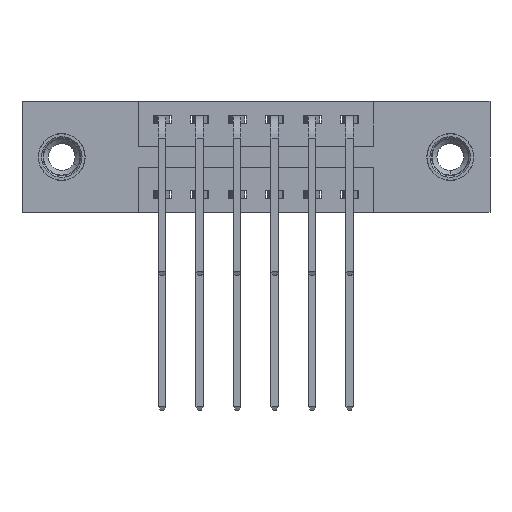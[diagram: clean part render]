
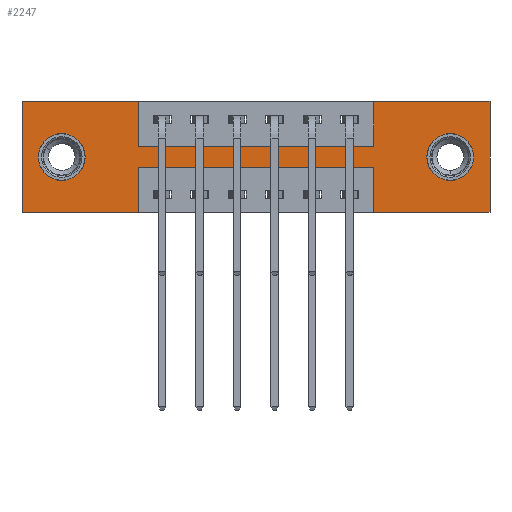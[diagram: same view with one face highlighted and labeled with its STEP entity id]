
A CAD part, front view. The second image highlights one B-rep face of the part: STEP entity #2247.
In plain terms, the highlighted planar face has unit normal (0, -1, 0).
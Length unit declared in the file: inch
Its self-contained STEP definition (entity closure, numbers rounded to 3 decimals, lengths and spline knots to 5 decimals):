
#42 = VERTEX_POINT ( 'NONE', #2623 ) ;
#102 = CARTESIAN_POINT ( 'NONE',  ( 1.4275, 0., -0.263 ) ) ;
#105 = ORIENTED_EDGE ( 'NONE', *, *, #3192, .F. ) ;
#121 = DIRECTION ( 'NONE',  ( 0., 0., -1. ) ) ;
#225 = CARTESIAN_POINT ( 'NONE',  ( 0., 0., 0. ) ) ;
#446 = CARTESIAN_POINT ( 'NONE',  ( 1.1725, 0., -0.37 ) ) ;
#526 = CARTESIAN_POINT ( 'NONE',  ( 0., 0., -0.37 ) ) ;
#544 = ORIENTED_EDGE ( 'NONE', *, *, #9212, .F. ) ;
#617 = ORIENTED_EDGE ( 'NONE', *, *, #5283, .F. ) ;
#626 = EDGE_CURVE ( 'NONE', #9823, #6591, #4002, .T. ) ;
#648 = VECTOR ( 'NONE', #1147, 39.37008 ) ;
#671 = AXIS2_PLACEMENT_3D ( 'NONE', #6473, #2868, #6435 ) ;
#1073 = DIRECTION ( 'NONE',  ( 1., 0., 0. ) ) ;
#1147 = DIRECTION ( 'NONE',  ( 0., 0., 1. ) ) ;
#1294 = EDGE_LOOP ( 'NONE', ( #617, #9598, #105, #4870, #7537, #4949, #3419, #544, #4352, #2203, #3891, #4409 ) ) ;
#1433 = CARTESIAN_POINT ( 'NONE',  ( 0.3875, 0., -0.37 ) ) ;
#1494 = LINE ( 'NONE', #11450, #3079 ) ;
#1506 = AXIS2_PLACEMENT_3D ( 'NONE', #7502, #6528, #4697 ) ;
#1885 = CARTESIAN_POINT ( 'NONE',  ( 0., 0., -0.37 ) ) ;
#2133 = AXIS2_PLACEMENT_3D ( 'NONE', #4694, #5673, #11016 ) ;
#2203 = ORIENTED_EDGE ( 'NONE', *, *, #8036, .F. ) ;
#2247 = ADVANCED_FACE ( 'NONE', ( #11677, #4725, #2288 ), #10993, .T. ) ;
#2263 = CARTESIAN_POINT ( 'NONE',  ( 0.3875, 0., -0.22 ) ) ;
#2288 = FACE_OUTER_BOUND ( 'NONE', #1294, .T. ) ;
#2499 = VECTOR ( 'NONE', #7907, 39.37008 ) ;
#2503 = LINE ( 'NONE', #5610, #10180 ) ;
#2623 = CARTESIAN_POINT ( 'NONE',  ( 0.1325, 0., -0.263 ) ) ;
#2700 = DIRECTION ( 'NONE',  ( 0., 1., 0. ) ) ;
#2743 = CARTESIAN_POINT ( 'NONE',  ( 0., 0., 0. ) ) ;
#2868 = DIRECTION ( 'NONE',  ( 0., 1., 0. ) ) ;
#2912 = VECTOR ( 'NONE', #4324, 39.37008 ) ;
#2934 = LINE ( 'NONE', #225, #8328 ) ;
#3079 = VECTOR ( 'NONE', #7864, 39.37008 ) ;
#3098 = AXIS2_PLACEMENT_3D ( 'NONE', #5759, #9308, #121 ) ;
#3192 = EDGE_CURVE ( 'NONE', #3302, #3218, #6525, .T. ) ;
#3218 = VERTEX_POINT ( 'NONE', #11252 ) ;
#3239 = CARTESIAN_POINT ( 'NONE',  ( 0.3875, 0., -0.15 ) ) ;
#3302 = VERTEX_POINT ( 'NONE', #446 ) ;
#3419 = ORIENTED_EDGE ( 'NONE', *, *, #11295, .F. ) ;
#3806 = CARTESIAN_POINT ( 'NONE',  ( 0.3875, 0., -0.37 ) ) ;
#3869 = CARTESIAN_POINT ( 'NONE',  ( 0.3875, 0., 0. ) ) ;
#3878 = EDGE_CURVE ( 'NONE', #4765, #9823, #5930, .T. ) ;
#3891 = ORIENTED_EDGE ( 'NONE', *, *, #626, .F. ) ;
#4002 = LINE ( 'NONE', #2743, #9795 ) ;
#4203 = CIRCLE ( 'NONE', #2133, 0.078 ) ;
#4206 = VERTEX_POINT ( 'NONE', #4833 ) ;
#4324 = DIRECTION ( 'NONE',  ( 0., 0., -1. ) ) ;
#4352 = ORIENTED_EDGE ( 'NONE', *, *, #11503, .F. ) ;
#4384 = CARTESIAN_POINT ( 'NONE',  ( 1.1725, 0., -0.15 ) ) ;
#4402 = CARTESIAN_POINT ( 'NONE',  ( 1.1725, 0., 0. ) ) ;
#4409 = ORIENTED_EDGE ( 'NONE', *, *, #3878, .F. ) ;
#4694 = CARTESIAN_POINT ( 'NONE',  ( 1.4275, 0., -0.185 ) ) ;
#4697 = DIRECTION ( 'NONE',  ( 0., 0., 1. ) ) ;
#4725 = FACE_BOUND ( 'NONE', #11133, .T. ) ;
#4765 = VERTEX_POINT ( 'NONE', #1433 ) ;
#4771 = CARTESIAN_POINT ( 'NONE',  ( 1.1725, 0., -0.37 ) ) ;
#4787 = DIRECTION ( 'NONE',  ( 1., 0., 0. ) ) ;
#4833 = CARTESIAN_POINT ( 'NONE',  ( 1.56, 0., 0. ) ) ;
#4870 = ORIENTED_EDGE ( 'NONE', *, *, #10159, .F. ) ;
#4912 = CIRCLE ( 'NONE', #9700, 0.078 ) ;
#4949 = ORIENTED_EDGE ( 'NONE', *, *, #6669, .F. ) ;
#5026 = VERTEX_POINT ( 'NONE', #2263 ) ;
#5088 = CARTESIAN_POINT ( 'NONE',  ( 0., 0., -0.37 ) ) ;
#5196 = DIRECTION ( 'NONE',  ( -1., 0., 0. ) ) ;
#5283 = EDGE_CURVE ( 'NONE', #5026, #4765, #7168, .T. ) ;
#5498 = VERTEX_POINT ( 'NONE', #3869 ) ;
#5610 = CARTESIAN_POINT ( 'NONE',  ( 0., 0., 0. ) ) ;
#5673 = DIRECTION ( 'NONE',  ( 0., 1., 0. ) ) ;
#5681 = CIRCLE ( 'NONE', #671, 0.078 ) ;
#5744 = VERTEX_POINT ( 'NONE', #6177 ) ;
#5759 = CARTESIAN_POINT ( 'NONE',  ( 0., 0., -0.37 ) ) ;
#5882 = EDGE_CURVE ( 'NONE', #42, #9236, #5681, .T. ) ;
#5930 = LINE ( 'NONE', #5088, #8997 ) ;
#6177 = CARTESIAN_POINT ( 'NONE',  ( 1.4275, 0., -0.107 ) ) ;
#6281 = ORIENTED_EDGE ( 'NONE', *, *, #11148, .T. ) ;
#6429 = DIRECTION ( 'NONE',  ( 0., 0., -1. ) ) ;
#6435 = DIRECTION ( 'NONE',  ( 0., 0., 1. ) ) ;
#6473 = CARTESIAN_POINT ( 'NONE',  ( 0.1325, 0., -0.185 ) ) ;
#6516 = DIRECTION ( 'NONE',  ( 1., 0., 0. ) ) ;
#6525 = LINE ( 'NONE', #4771, #648 ) ;
#6528 = DIRECTION ( 'NONE',  ( 0., 1., 0. ) ) ;
#6591 = VERTEX_POINT ( 'NONE', #11084 ) ;
#6669 = EDGE_CURVE ( 'NONE', #7861, #4206, #2503, .T. ) ;
#6764 = VECTOR ( 'NONE', #1073, 39.37008 ) ;
#6788 = LINE ( 'NONE', #9755, #2912 ) ;
#6882 = EDGE_CURVE ( 'NONE', #4206, #8944, #1494, .T. ) ;
#7168 = LINE ( 'NONE', #3806, #9129 ) ;
#7307 = LINE ( 'NONE', #9394, #6764 ) ;
#7467 = EDGE_CURVE ( 'NONE', #3218, #5026, #11259, .T. ) ;
#7502 = CARTESIAN_POINT ( 'NONE',  ( 0.1325, 0., -0.185 ) ) ;
#7537 = ORIENTED_EDGE ( 'NONE', *, *, #6882, .F. ) ;
#7637 = DIRECTION ( 'NONE',  ( -1., 0., 0. ) ) ;
#7759 = VECTOR ( 'NONE', #10103, 39.37008 ) ;
#7861 = VERTEX_POINT ( 'NONE', #4402 ) ;
#7864 = DIRECTION ( 'NONE',  ( 0., 0., -1. ) ) ;
#7907 = DIRECTION ( 'NONE',  ( -1., 0., 0. ) ) ;
#7977 = EDGE_CURVE ( 'NONE', #5744, #11000, #4203, .T. ) ;
#8003 = CIRCLE ( 'NONE', #1506, 0.078 ) ;
#8036 = EDGE_CURVE ( 'NONE', #6591, #5498, #2934, .T. ) ;
#8135 = CARTESIAN_POINT ( 'NONE',  ( 1.4275, 0., -0.185 ) ) ;
#8287 = VERTEX_POINT ( 'NONE', #3239 ) ;
#8302 = LINE ( 'NONE', #10957, #7759 ) ;
#8328 = VECTOR ( 'NONE', #4787, 39.37008 ) ;
#8647 = CARTESIAN_POINT ( 'NONE',  ( 0.1325, 0., -0.107 ) ) ;
#8674 = CARTESIAN_POINT ( 'NONE',  ( 0.3875, 0., -0.22 ) ) ;
#8944 = VERTEX_POINT ( 'NONE', #10031 ) ;
#8977 = ORIENTED_EDGE ( 'NONE', *, *, #11665, .T. ) ;
#8997 = VECTOR ( 'NONE', #5196, 39.37008 ) ;
#9095 = DIRECTION ( 'NONE',  ( 0., 0., 1. ) ) ;
#9129 = VECTOR ( 'NONE', #10157, 39.37008 ) ;
#9212 = EDGE_CURVE ( 'NONE', #8287, #9526, #7307, .T. ) ;
#9236 = VERTEX_POINT ( 'NONE', #8647 ) ;
#9308 = DIRECTION ( 'NONE',  ( 0., -1., 0. ) ) ;
#9394 = CARTESIAN_POINT ( 'NONE',  ( 0.3875, 0., -0.15 ) ) ;
#9526 = VERTEX_POINT ( 'NONE', #4384 ) ;
#9598 = ORIENTED_EDGE ( 'NONE', *, *, #7467, .F. ) ;
#9700 = AXIS2_PLACEMENT_3D ( 'NONE', #8135, #2700, #6429 ) ;
#9731 = LINE ( 'NONE', #526, #2499 ) ;
#9755 = CARTESIAN_POINT ( 'NONE',  ( 0.3875, 0., 0. ) ) ;
#9795 = VECTOR ( 'NONE', #9095, 39.37008 ) ;
#9823 = VERTEX_POINT ( 'NONE', #1885 ) ;
#10031 = CARTESIAN_POINT ( 'NONE',  ( 1.56, 0., -0.37 ) ) ;
#10103 = DIRECTION ( 'NONE',  ( 0., 0., 1. ) ) ;
#10105 = VECTOR ( 'NONE', #7637, 39.37008 ) ;
#10157 = DIRECTION ( 'NONE',  ( 0., 0., -1. ) ) ;
#10159 = EDGE_CURVE ( 'NONE', #8944, #3302, #9731, .T. ) ;
#10180 = VECTOR ( 'NONE', #6516, 39.37008 ) ;
#10319 = ORIENTED_EDGE ( 'NONE', *, *, #7977, .T. ) ;
#10957 = CARTESIAN_POINT ( 'NONE',  ( 1.1725, 0., 0. ) ) ;
#10993 = PLANE ( 'NONE',  #3098 ) ;
#11000 = VERTEX_POINT ( 'NONE', #102 ) ;
#11016 = DIRECTION ( 'NONE',  ( 0., 0., -1. ) ) ;
#11084 = CARTESIAN_POINT ( 'NONE',  ( 0., 0., 0. ) ) ;
#11133 = EDGE_LOOP ( 'NONE', ( #8977, #11457 ) ) ;
#11148 = EDGE_CURVE ( 'NONE', #11000, #5744, #4912, .T. ) ;
#11252 = CARTESIAN_POINT ( 'NONE',  ( 1.1725, 0., -0.22 ) ) ;
#11259 = LINE ( 'NONE', #8674, #10105 ) ;
#11295 = EDGE_CURVE ( 'NONE', #9526, #7861, #8302, .T. ) ;
#11409 = EDGE_LOOP ( 'NONE', ( #10319, #6281 ) ) ;
#11450 = CARTESIAN_POINT ( 'NONE',  ( 1.56, 0., 0. ) ) ;
#11457 = ORIENTED_EDGE ( 'NONE', *, *, #5882, .T. ) ;
#11503 = EDGE_CURVE ( 'NONE', #5498, #8287, #6788, .T. ) ;
#11665 = EDGE_CURVE ( 'NONE', #9236, #42, #8003, .T. ) ;
#11677 = FACE_BOUND ( 'NONE', #11409, .T. ) ;
